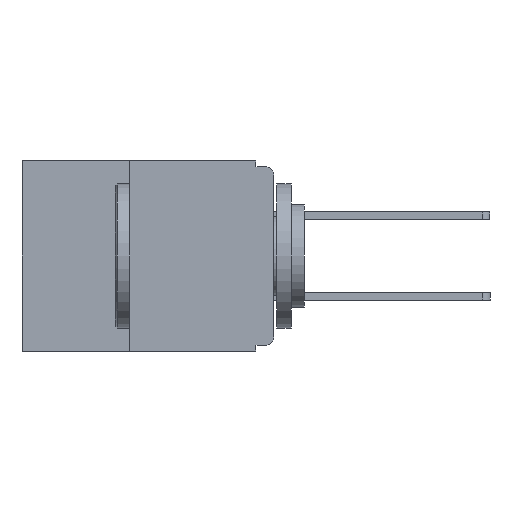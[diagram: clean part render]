
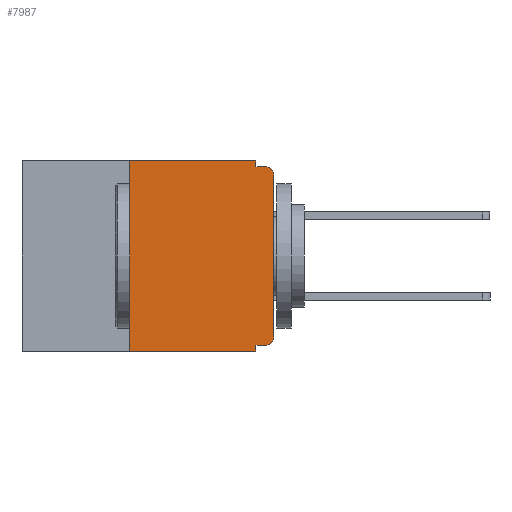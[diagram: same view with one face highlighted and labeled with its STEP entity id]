
A CAD part, left-side view. The second image highlights one B-rep face of the part: STEP entity #7987.
In plain terms, the highlighted planar face has unit normal (-1, 0, 0).
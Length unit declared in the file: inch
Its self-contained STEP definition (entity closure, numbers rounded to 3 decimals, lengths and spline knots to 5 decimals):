
#234 = CARTESIAN_POINT ( 'NONE',  ( 0., 0.031, -0.32 ) ) ;
#369 = ORIENTED_EDGE ( 'NONE', *, *, #25539, .T. ) ;
#1179 = LINE ( 'NONE', #8445, #27192 ) ;
#1253 = DIRECTION ( 'NONE',  ( -1., 0., 0. ) ) ;
#1339 = CARTESIAN_POINT ( 'NONE',  ( 0., 0.031, 0. ) ) ;
#1935 = ORIENTED_EDGE ( 'NONE', *, *, #6963, .F. ) ;
#2069 = VERTEX_POINT ( 'NONE', #10230 ) ;
#2406 = DIRECTION ( 'NONE',  ( 0., 0., -1. ) ) ;
#2589 = EDGE_CURVE ( 'NONE', #26950, #30337, #16937, .T. ) ;
#3056 = VERTEX_POINT ( 'NONE', #3697 ) ;
#3308 = CARTESIAN_POINT ( 'NONE',  ( 0., 0.015, -0.01 ) ) ;
#3467 = ORIENTED_EDGE ( 'NONE', *, *, #19301, .T. ) ;
#3697 = CARTESIAN_POINT ( 'NONE',  ( 0., 0., -0.025 ) ) ;
#4094 = VECTOR ( 'NONE', #14528, 39.37008 ) ;
#4388 = CARTESIAN_POINT ( 'NONE',  ( 0., 0.031, 0. ) ) ;
#4892 = LINE ( 'NONE', #22045, #4094 ) ;
#4988 = CARTESIAN_POINT ( 'NONE',  ( 0., 0.031, -0.33 ) ) ;
#5604 = CARTESIAN_POINT ( 'NONE',  ( 0., 0.031, -0.01 ) ) ;
#6673 = DIRECTION ( 'NONE',  ( -1., 0., 0. ) ) ;
#6946 = DIRECTION ( 'NONE',  ( 0., 0., -1. ) ) ;
#6963 = EDGE_CURVE ( 'NONE', #26067, #8345, #4892, .T. ) ;
#7685 = CARTESIAN_POINT ( 'NONE',  ( 0., 0.015, -0.32 ) ) ;
#7987 = ADVANCED_FACE ( 'NONE', ( #13558 ), #23380, .F. ) ;
#8345 = VERTEX_POINT ( 'NONE', #22699 ) ;
#8445 = CARTESIAN_POINT ( 'NONE',  ( 0., 0., -0.32 ) ) ;
#8500 = EDGE_CURVE ( 'NONE', #8345, #20051, #15451, .T. ) ;
#8526 = EDGE_CURVE ( 'NONE', #10203, #32190, #1179, .T. ) ;
#8740 = VECTOR ( 'NONE', #10919, 39.37008 ) ;
#9145 = CARTESIAN_POINT ( 'NONE',  ( 0., 0., -0.01 ) ) ;
#9376 = CIRCLE ( 'NONE', #22791, 0.015 ) ;
#9564 = LINE ( 'NONE', #25319, #27994 ) ;
#10036 = LINE ( 'NONE', #21841, #29209 ) ;
#10203 = VERTEX_POINT ( 'NONE', #7685 ) ;
#10230 = CARTESIAN_POINT ( 'NONE',  ( 0., 0., -0.305 ) ) ;
#10338 = DIRECTION ( 'NONE',  ( 0., 0., 1. ) ) ;
#10919 = DIRECTION ( 'NONE',  ( 0., -1., 0. ) ) ;
#11140 = ORIENTED_EDGE ( 'NONE', *, *, #8526, .F. ) ;
#11913 = DIRECTION ( 'NONE',  ( 0., -1., 0. ) ) ;
#13224 = EDGE_LOOP ( 'NONE', ( #3467, #25737, #25716, #14838, #23879, #1935, #369, #17121, #11140, #18820 ) ) ;
#13466 = DIRECTION ( 'NONE',  ( 1., 0., 0. ) ) ;
#13558 = FACE_OUTER_BOUND ( 'NONE', #13224, .T. ) ;
#13636 = AXIS2_PLACEMENT_3D ( 'NONE', #28436, #13466, #30837 ) ;
#14113 = CARTESIAN_POINT ( 'NONE',  ( 0., 0.031, -0.33 ) ) ;
#14528 = DIRECTION ( 'NONE',  ( 0., 0., 1. ) ) ;
#14537 = VERTEX_POINT ( 'NONE', #14113 ) ;
#14838 = ORIENTED_EDGE ( 'NONE', *, *, #24356, .F. ) ;
#15451 = LINE ( 'NONE', #25779, #8740 ) ;
#16249 = EDGE_CURVE ( 'NONE', #3056, #30337, #29444, .T. ) ;
#16420 = CARTESIAN_POINT ( 'NONE',  ( 0., 0.015, -0.025 ) ) ;
#16739 = LINE ( 'NONE', #4388, #29218 ) ;
#16937 = LINE ( 'NONE', #9145, #20422 ) ;
#17121 = ORIENTED_EDGE ( 'NONE', *, *, #22238, .F. ) ;
#18820 = ORIENTED_EDGE ( 'NONE', *, *, #21992, .T. ) ;
#18912 = DIRECTION ( 'NONE',  ( 0., 0., -1. ) ) ;
#19301 = EDGE_CURVE ( 'NONE', #2069, #3056, #9564, .T. ) ;
#20051 = VERTEX_POINT ( 'NONE', #1339 ) ;
#20304 = DIRECTION ( 'NONE',  ( 0., -1., 0. ) ) ;
#20422 = VECTOR ( 'NONE', #20304, 39.37008 ) ;
#20723 = VECTOR ( 'NONE', #2406, 39.37008 ) ;
#21728 = CARTESIAN_POINT ( 'NONE',  ( 0., 0.015, -0.305 ) ) ;
#21841 = CARTESIAN_POINT ( 'NONE',  ( 0., 0.437, -0.33 ) ) ;
#21992 = EDGE_CURVE ( 'NONE', #10203, #2069, #9376, .T. ) ;
#22045 = CARTESIAN_POINT ( 'NONE',  ( 0., 0.25, -0.33 ) ) ;
#22238 = EDGE_CURVE ( 'NONE', #32190, #14537, #27390, .T. ) ;
#22699 = CARTESIAN_POINT ( 'NONE',  ( 0., 0.25, 0. ) ) ;
#22791 = AXIS2_PLACEMENT_3D ( 'NONE', #21728, #6673, #24229 ) ;
#23380 = PLANE ( 'NONE',  #13636 ) ;
#23879 = ORIENTED_EDGE ( 'NONE', *, *, #8500, .F. ) ;
#24229 = DIRECTION ( 'NONE',  ( 0., 0., -1. ) ) ;
#24356 = EDGE_CURVE ( 'NONE', #20051, #26950, #16739, .T. ) ;
#25319 = CARTESIAN_POINT ( 'NONE',  ( 0., 0., 0. ) ) ;
#25539 = EDGE_CURVE ( 'NONE', #26067, #14537, #10036, .T. ) ;
#25716 = ORIENTED_EDGE ( 'NONE', *, *, #2589, .F. ) ;
#25737 = ORIENTED_EDGE ( 'NONE', *, *, #16249, .T. ) ;
#25741 = AXIS2_PLACEMENT_3D ( 'NONE', #16420, #1253, #18912 ) ;
#25779 = CARTESIAN_POINT ( 'NONE',  ( 0., 0.437, 0. ) ) ;
#26067 = VERTEX_POINT ( 'NONE', #29837 ) ;
#26950 = VERTEX_POINT ( 'NONE', #5604 ) ;
#27192 = VECTOR ( 'NONE', #30921, 39.37008 ) ;
#27390 = LINE ( 'NONE', #4988, #20723 ) ;
#27994 = VECTOR ( 'NONE', #10338, 39.37008 ) ;
#28436 = CARTESIAN_POINT ( 'NONE',  ( 0., 0.437, 0. ) ) ;
#29209 = VECTOR ( 'NONE', #11913, 39.37008 ) ;
#29218 = VECTOR ( 'NONE', #6946, 39.37008 ) ;
#29444 = CIRCLE ( 'NONE', #25741, 0.015 ) ;
#29837 = CARTESIAN_POINT ( 'NONE',  ( 0., 0.25, -0.33 ) ) ;
#30337 = VERTEX_POINT ( 'NONE', #3308 ) ;
#30837 = DIRECTION ( 'NONE',  ( 0., 0., -1. ) ) ;
#30921 = DIRECTION ( 'NONE',  ( 0., 1., 0. ) ) ;
#32190 = VERTEX_POINT ( 'NONE', #234 ) ;
